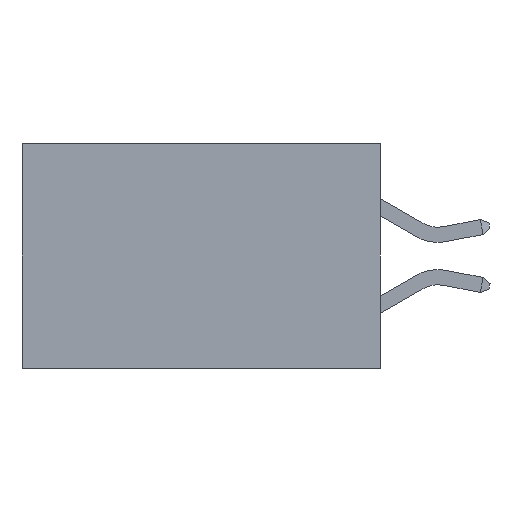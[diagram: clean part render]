
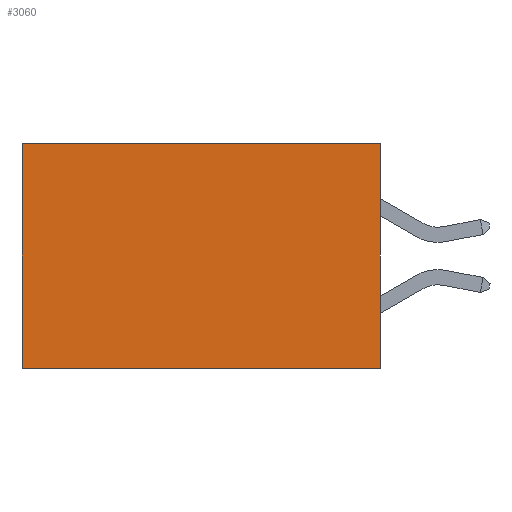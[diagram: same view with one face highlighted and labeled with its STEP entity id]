
A CAD part, left-side view. The second image highlights one B-rep face of the part: STEP entity #3060.
In plain terms, the highlighted planar face has unit normal (-1, 0, 0).
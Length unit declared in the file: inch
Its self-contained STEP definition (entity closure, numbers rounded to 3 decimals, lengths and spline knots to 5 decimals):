
#327 = CARTESIAN_POINT ( 'NONE',  ( 0.277, 0.59, -0.37 ) ) ;
#695 = EDGE_CURVE ( 'NONE', #2744, #7273, #5712, .T. ) ;
#1133 = VECTOR ( 'NONE', #3595, 39.37008 ) ;
#1280 = VECTOR ( 'NONE', #2818, 39.37008 ) ;
#1602 = LINE ( 'NONE', #10639, #1280 ) ;
#2098 = EDGE_CURVE ( 'NONE', #3083, #7273, #2964, .T. ) ;
#2744 = VERTEX_POINT ( 'NONE', #11371 ) ;
#2818 = DIRECTION ( 'NONE',  ( 0., 1., 0. ) ) ;
#2964 = LINE ( 'NONE', #327, #7474 ) ;
#2999 = VECTOR ( 'NONE', #3149, 39.37008 ) ;
#3060 = ADVANCED_FACE ( 'NONE', ( #11051 ), #11072, .F. ) ;
#3083 = VERTEX_POINT ( 'NONE', #10039 ) ;
#3149 = DIRECTION ( 'NONE',  ( 0., 1., 0. ) ) ;
#3595 = DIRECTION ( 'NONE',  ( 0., 0., -1. ) ) ;
#4183 = DIRECTION ( 'NONE',  ( 0., 0., -1. ) ) ;
#4650 = ORIENTED_EDGE ( 'NONE', *, *, #2098, .T. ) ;
#4687 = ORIENTED_EDGE ( 'NONE', *, *, #695, .F. ) ;
#4716 = ORIENTED_EDGE ( 'NONE', *, *, #10351, .F. ) ;
#4730 = ORIENTED_EDGE ( 'NONE', *, *, #10601, .T. ) ;
#5712 = LINE ( 'NONE', #9413, #2999 ) ;
#7273 = VERTEX_POINT ( 'NONE', #11283 ) ;
#7474 = VECTOR ( 'NONE', #4183, 39.37008 ) ;
#8263 = LINE ( 'NONE', #8800, #1133 ) ;
#8800 = CARTESIAN_POINT ( 'NONE',  ( 0.277, 0., -0.37 ) ) ;
#9249 = CARTESIAN_POINT ( 'NONE',  ( 0.277, 0., 0. ) ) ;
#9413 = CARTESIAN_POINT ( 'NONE',  ( 0.277, 0., -0.37 ) ) ;
#10039 = CARTESIAN_POINT ( 'NONE',  ( 0.277, 0.59, 0. ) ) ;
#10351 = EDGE_CURVE ( 'NONE', #10813, #2744, #8263, .T. ) ;
#10599 = DIRECTION ( 'NONE',  ( 0., 0., -1. ) ) ;
#10601 = EDGE_CURVE ( 'NONE', #10813, #3083, #1602, .T. ) ;
#10639 = CARTESIAN_POINT ( 'NONE',  ( 0.277, 0., 0. ) ) ;
#10663 = DIRECTION ( 'NONE',  ( 1., 0., 0. ) ) ;
#10795 = EDGE_LOOP ( 'NONE', ( #4650, #4687, #4716, #4730 ) ) ;
#10813 = VERTEX_POINT ( 'NONE', #9249 ) ;
#10875 = CARTESIAN_POINT ( 'NONE',  ( 0.277, 0., -0.37 ) ) ;
#11047 = AXIS2_PLACEMENT_3D ( 'NONE', #10875, #10663, #10599 ) ;
#11051 = FACE_OUTER_BOUND ( 'NONE', #10795, .T. ) ;
#11072 = PLANE ( 'NONE',  #11047 ) ;
#11283 = CARTESIAN_POINT ( 'NONE',  ( 0.277, 0.59, -0.37 ) ) ;
#11371 = CARTESIAN_POINT ( 'NONE',  ( 0.277, 0., -0.37 ) ) ;
